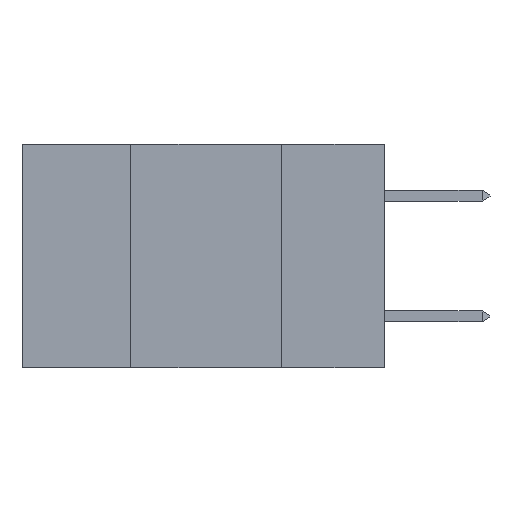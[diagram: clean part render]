
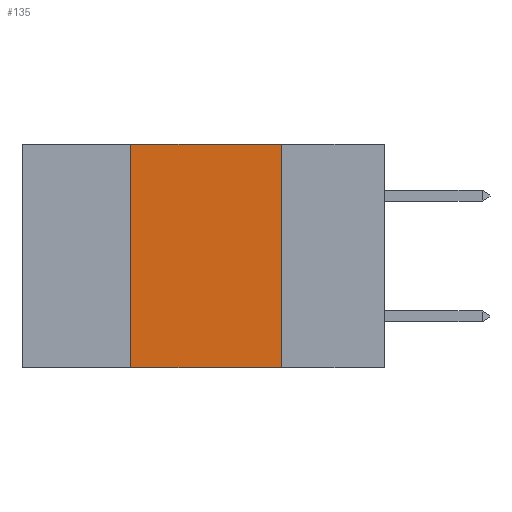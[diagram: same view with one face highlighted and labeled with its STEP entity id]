
A CAD part, left-side view. The second image highlights one B-rep face of the part: STEP entity #135.
In plain terms, the highlighted planar face has unit normal (-1, 0, 0).
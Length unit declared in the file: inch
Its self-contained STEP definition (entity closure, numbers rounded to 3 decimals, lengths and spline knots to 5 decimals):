
#135 = ADVANCED_FACE ( 'NONE', ( #1036 ), #4944, .F. ) ;
#200 = DIRECTION ( 'NONE',  ( 0., -1., 0. ) ) ;
#332 = VECTOR ( 'NONE', #9013, 39.37008 ) ;
#411 = DIRECTION ( 'NONE',  ( 0., -1., 0. ) ) ;
#525 = CARTESIAN_POINT ( 'NONE',  ( 0., 0.17, 0. ) ) ;
#568 = AXIS2_PLACEMENT_3D ( 'NONE', #2080, #2160, #7917 ) ;
#1036 = FACE_OUTER_BOUND ( 'NONE', #10282, .T. ) ;
#1265 = CARTESIAN_POINT ( 'NONE',  ( 0., 0.42, 0. ) ) ;
#1505 = ORIENTED_EDGE ( 'NONE', *, *, #6682, .F. ) ;
#2080 = CARTESIAN_POINT ( 'NONE',  ( 0., 0.6, 0. ) ) ;
#2160 = DIRECTION ( 'NONE',  ( 1., 0., 0. ) ) ;
#2326 = LINE ( 'NONE', #10237, #5492 ) ;
#2728 = ORIENTED_EDGE ( 'NONE', *, *, #10170, .F. ) ;
#3389 = LINE ( 'NONE', #12208, #11114 ) ;
#3526 = EDGE_CURVE ( 'NONE', #6319, #8986, #2326, .T. ) ;
#4279 = LINE ( 'NONE', #1265, #332 ) ;
#4396 = DIRECTION ( 'NONE',  ( 0., 0., -1. ) ) ;
#4854 = VERTEX_POINT ( 'NONE', #10314 ) ;
#4944 = PLANE ( 'NONE',  #568 ) ;
#4984 = CARTESIAN_POINT ( 'NONE',  ( 0., 0.17, -0.37 ) ) ;
#5492 = VECTOR ( 'NONE', #4396, 39.37008 ) ;
#6168 = EDGE_CURVE ( 'NONE', #10908, #8986, #3389, .T. ) ;
#6319 = VERTEX_POINT ( 'NONE', #525 ) ;
#6682 = EDGE_CURVE ( 'NONE', #10908, #4854, #4279, .T. ) ;
#6986 = CARTESIAN_POINT ( 'NONE',  ( 0., 0.42, -0.37 ) ) ;
#7179 = VECTOR ( 'NONE', #411, 39.37008 ) ;
#7917 = DIRECTION ( 'NONE',  ( 0., 0., -1. ) ) ;
#8393 = CARTESIAN_POINT ( 'NONE',  ( 0., 0.6, 0. ) ) ;
#8986 = VERTEX_POINT ( 'NONE', #4984 ) ;
#9013 = DIRECTION ( 'NONE',  ( 0., 0., 1. ) ) ;
#9370 = ORIENTED_EDGE ( 'NONE', *, *, #6168, .T. ) ;
#10170 = EDGE_CURVE ( 'NONE', #4854, #6319, #10488, .T. ) ;
#10237 = CARTESIAN_POINT ( 'NONE',  ( 0., 0.17, 0. ) ) ;
#10282 = EDGE_LOOP ( 'NONE', ( #10485, #2728, #1505, #9370 ) ) ;
#10314 = CARTESIAN_POINT ( 'NONE',  ( 0., 0.42, 0. ) ) ;
#10485 = ORIENTED_EDGE ( 'NONE', *, *, #3526, .F. ) ;
#10488 = LINE ( 'NONE', #8393, #7179 ) ;
#10908 = VERTEX_POINT ( 'NONE', #6986 ) ;
#11114 = VECTOR ( 'NONE', #200, 39.37008 ) ;
#12208 = CARTESIAN_POINT ( 'NONE',  ( 0., 0.6, -0.37 ) ) ;
